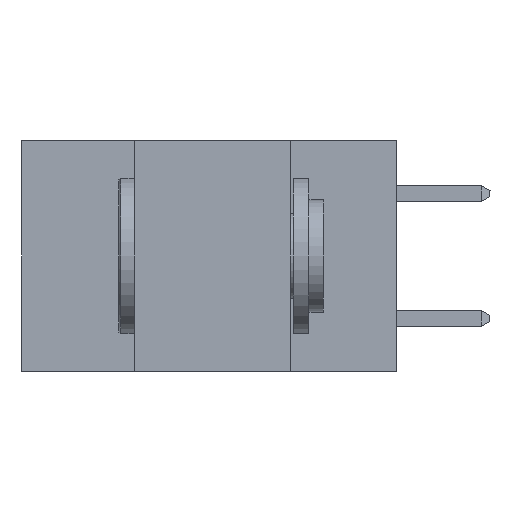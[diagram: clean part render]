
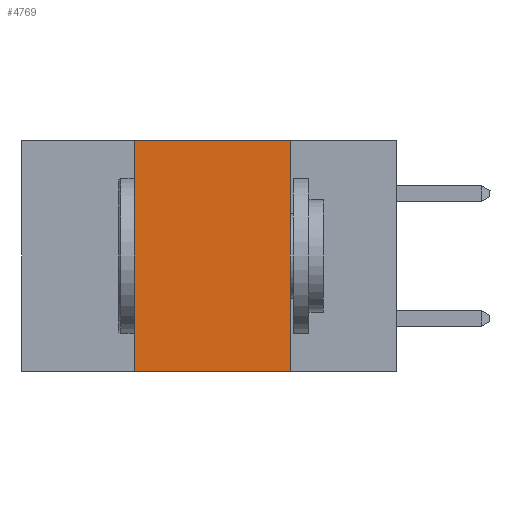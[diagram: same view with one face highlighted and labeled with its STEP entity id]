
A CAD part, left-side view. The second image highlights one B-rep face of the part: STEP entity #4769.
In plain terms, the highlighted planar face has unit normal (-1, 0, 0).
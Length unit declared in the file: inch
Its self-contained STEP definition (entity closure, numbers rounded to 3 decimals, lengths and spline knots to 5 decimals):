
#464 = VERTEX_POINT ( 'NONE', #5083 ) ;
#759 = VERTEX_POINT ( 'NONE', #8810 ) ;
#1585 = LINE ( 'NONE', #4809, #4843 ) ;
#2062 = DIRECTION ( 'NONE',  ( 0., 0., -1. ) ) ;
#2306 = ORIENTED_EDGE ( 'NONE', *, *, #16731, .F. ) ;
#2449 = EDGE_LOOP ( 'NONE', ( #2306, #7796, #16525, #5484 ) ) ;
#2883 = VERTEX_POINT ( 'NONE', #11005 ) ;
#4769 = ADVANCED_FACE ( 'NONE', ( #12422 ), #12970, .F. ) ;
#4809 = CARTESIAN_POINT ( 'NONE',  ( 0., 0.17, 0. ) ) ;
#4843 = VECTOR ( 'NONE', #2062, 39.37008 ) ;
#5083 = CARTESIAN_POINT ( 'NONE',  ( 0., 0.17, -0.37 ) ) ;
#5484 = ORIENTED_EDGE ( 'NONE', *, *, #16776, .T. ) ;
#5564 = AXIS2_PLACEMENT_3D ( 'NONE', #10339, #15523, #7727 ) ;
#6303 = DIRECTION ( 'NONE',  ( 0., 0., 1. ) ) ;
#7424 = VECTOR ( 'NONE', #14847, 39.37008 ) ;
#7727 = DIRECTION ( 'NONE',  ( 0., 0., -1. ) ) ;
#7780 = CARTESIAN_POINT ( 'NONE',  ( 0., 0.6, -0.37 ) ) ;
#7796 = ORIENTED_EDGE ( 'NONE', *, *, #9137, .F. ) ;
#8810 = CARTESIAN_POINT ( 'NONE',  ( 0., 0.17, 0. ) ) ;
#9135 = DIRECTION ( 'NONE',  ( 0., -1., 0. ) ) ;
#9137 = EDGE_CURVE ( 'NONE', #2883, #759, #10975, .T. ) ;
#9636 = CARTESIAN_POINT ( 'NONE',  ( 0., 0.6, 0. ) ) ;
#10339 = CARTESIAN_POINT ( 'NONE',  ( 0., 0.6, 0. ) ) ;
#10772 = LINE ( 'NONE', #7780, #17160 ) ;
#10975 = LINE ( 'NONE', #9636, #7424 ) ;
#11005 = CARTESIAN_POINT ( 'NONE',  ( 0., 0.42, 0. ) ) ;
#12422 = FACE_OUTER_BOUND ( 'NONE', #2449, .T. ) ;
#12970 = PLANE ( 'NONE',  #5564 ) ;
#14219 = CARTESIAN_POINT ( 'NONE',  ( 0., 0.42, 0. ) ) ;
#14615 = LINE ( 'NONE', #14219, #15005 ) ;
#14847 = DIRECTION ( 'NONE',  ( 0., -1., 0. ) ) ;
#15005 = VECTOR ( 'NONE', #6303, 39.37008 ) ;
#15035 = VERTEX_POINT ( 'NONE', #16218 ) ;
#15523 = DIRECTION ( 'NONE',  ( 1., 0., 0. ) ) ;
#16218 = CARTESIAN_POINT ( 'NONE',  ( 0., 0.42, -0.37 ) ) ;
#16525 = ORIENTED_EDGE ( 'NONE', *, *, #16756, .F. ) ;
#16731 = EDGE_CURVE ( 'NONE', #759, #464, #1585, .T. ) ;
#16756 = EDGE_CURVE ( 'NONE', #15035, #2883, #14615, .T. ) ;
#16776 = EDGE_CURVE ( 'NONE', #15035, #464, #10772, .T. ) ;
#17160 = VECTOR ( 'NONE', #9135, 39.37008 ) ;
